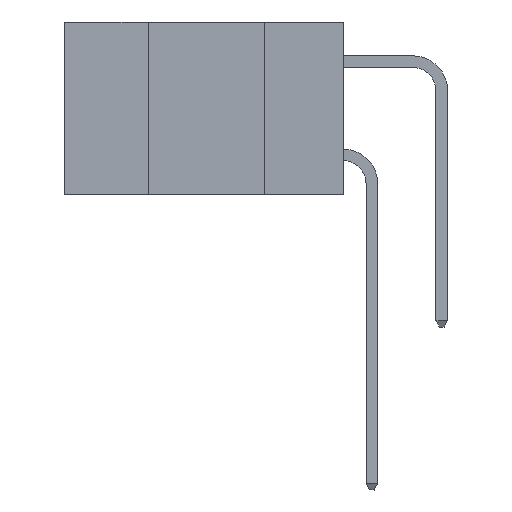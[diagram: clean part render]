
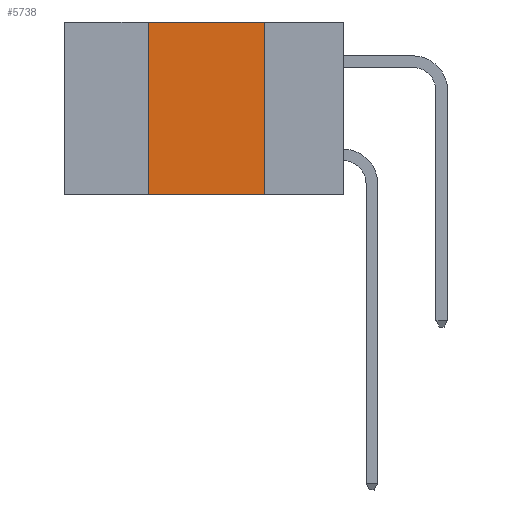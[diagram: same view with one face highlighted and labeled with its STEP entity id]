
A CAD part, left-side view. The second image highlights one B-rep face of the part: STEP entity #5738.
In plain terms, the highlighted planar face has unit normal (-1, 0, 0).
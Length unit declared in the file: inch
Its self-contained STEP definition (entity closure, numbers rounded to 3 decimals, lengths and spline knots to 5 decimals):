
#231 = LINE ( 'NONE', #10722, #16316 ) ;
#402 = VERTEX_POINT ( 'NONE', #6799 ) ;
#1681 = VERTEX_POINT ( 'NONE', #13271 ) ;
#2030 = DIRECTION ( 'NONE',  ( 0., -1., 0. ) ) ;
#2812 = CARTESIAN_POINT ( 'NONE',  ( 0., 0.6, -0.37 ) ) ;
#2976 = ORIENTED_EDGE ( 'NONE', *, *, #4218, .F. ) ;
#3130 = VECTOR ( 'NONE', #4010, 39.37008 ) ;
#3323 = EDGE_CURVE ( 'NONE', #1681, #15107, #10066, .T. ) ;
#3576 = VECTOR ( 'NONE', #2030, 39.37008 ) ;
#4010 = DIRECTION ( 'NONE',  ( 0., 0., 1. ) ) ;
#4218 = EDGE_CURVE ( 'NONE', #1681, #8350, #13631, .T. ) ;
#4362 = DIRECTION ( 'NONE',  ( 1., 0., 0. ) ) ;
#4662 = PLANE ( 'NONE',  #5993 ) ;
#4746 = DIRECTION ( 'NONE',  ( 0., -1., 0. ) ) ;
#5208 = LINE ( 'NONE', #7305, #14729 ) ;
#5738 = ADVANCED_FACE ( 'NONE', ( #13705 ), #4662, .F. ) ;
#5991 = EDGE_CURVE ( 'NONE', #402, #15107, #231, .T. ) ;
#5993 = AXIS2_PLACEMENT_3D ( 'NONE', #12731, #4362, #12091 ) ;
#6408 = DIRECTION ( 'NONE',  ( 0., 0., -1. ) ) ;
#6695 = CARTESIAN_POINT ( 'NONE',  ( 0., 0.42, 0. ) ) ;
#6799 = CARTESIAN_POINT ( 'NONE',  ( 0., 0.17, 0. ) ) ;
#6930 = CARTESIAN_POINT ( 'NONE',  ( 0., 0.17, -0.37 ) ) ;
#7302 = EDGE_CURVE ( 'NONE', #8350, #402, #5208, .T. ) ;
#7305 = CARTESIAN_POINT ( 'NONE',  ( 0., 0.6, 0. ) ) ;
#8350 = VERTEX_POINT ( 'NONE', #15377 ) ;
#9081 = ORIENTED_EDGE ( 'NONE', *, *, #5991, .F. ) ;
#9493 = ORIENTED_EDGE ( 'NONE', *, *, #7302, .F. ) ;
#9886 = ORIENTED_EDGE ( 'NONE', *, *, #3323, .T. ) ;
#10066 = LINE ( 'NONE', #2812, #3576 ) ;
#10722 = CARTESIAN_POINT ( 'NONE',  ( 0., 0.17, 0. ) ) ;
#12091 = DIRECTION ( 'NONE',  ( 0., 0., -1. ) ) ;
#12404 = EDGE_LOOP ( 'NONE', ( #9081, #9493, #2976, #9886 ) ) ;
#12731 = CARTESIAN_POINT ( 'NONE',  ( 0., 0.6, 0. ) ) ;
#13271 = CARTESIAN_POINT ( 'NONE',  ( 0., 0.42, -0.37 ) ) ;
#13631 = LINE ( 'NONE', #6695, #3130 ) ;
#13705 = FACE_OUTER_BOUND ( 'NONE', #12404, .T. ) ;
#14729 = VECTOR ( 'NONE', #4746, 39.37008 ) ;
#15107 = VERTEX_POINT ( 'NONE', #6930 ) ;
#15377 = CARTESIAN_POINT ( 'NONE',  ( 0., 0.42, 0. ) ) ;
#16316 = VECTOR ( 'NONE', #6408, 39.37008 ) ;
